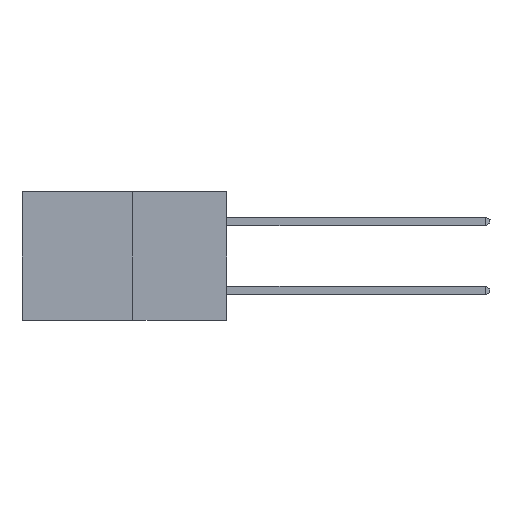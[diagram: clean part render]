
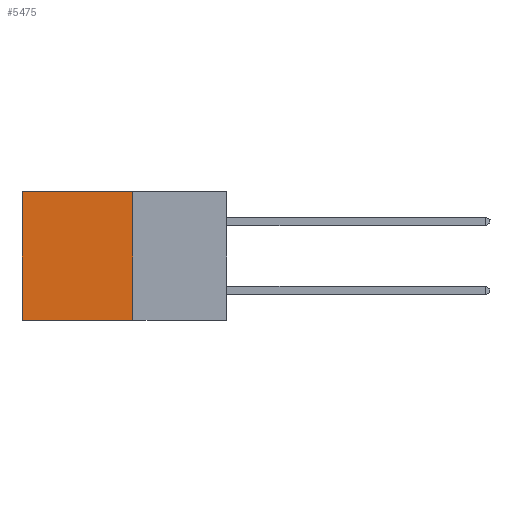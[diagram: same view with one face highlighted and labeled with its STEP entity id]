
A CAD part, left-side view. The second image highlights one B-rep face of the part: STEP entity #5475.
In plain terms, the highlighted planar face has unit normal (-1, 0, 0).
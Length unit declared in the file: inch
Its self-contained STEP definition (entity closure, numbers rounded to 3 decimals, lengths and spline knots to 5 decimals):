
#87 = AXIS2_PLACEMENT_3D ( 'NONE', #12365, #12074, #12022 ) ;
#918 = CARTESIAN_POINT ( 'NONE',  ( 0.277, 0.27, -0.37 ) ) ;
#1489 = CARTESIAN_POINT ( 'NONE',  ( 0.277, 0.27, 0. ) ) ;
#1579 = VERTEX_POINT ( 'NONE', #26224 ) ;
#1905 = ORIENTED_EDGE ( 'NONE', *, *, #10503, .T. ) ;
#2034 = FACE_OUTER_BOUND ( 'NONE', #7425, .T. ) ;
#2120 = CARTESIAN_POINT ( 'NONE',  ( 0.277, 0.27, -0.37 ) ) ;
#5475 = ADVANCED_FACE ( 'NONE', ( #2034 ), #12141, .F. ) ;
#6889 = LINE ( 'NONE', #16978, #12158 ) ;
#7425 = EDGE_LOOP ( 'NONE', ( #1905, #21946, #28570, #7823 ) ) ;
#7705 = CARTESIAN_POINT ( 'NONE',  ( 0.277, 0.59, -0.37 ) ) ;
#7823 = ORIENTED_EDGE ( 'NONE', *, *, #11074, .T. ) ;
#9882 = LINE ( 'NONE', #2120, #15215 ) ;
#10503 = EDGE_CURVE ( 'NONE', #19440, #12695, #6889, .T. ) ;
#11074 = EDGE_CURVE ( 'NONE', #1579, #19440, #13713, .T. ) ;
#11922 = DIRECTION ( 'NONE',  ( 0., 0., -1. ) ) ;
#12022 = DIRECTION ( 'NONE',  ( 0., 0., -1. ) ) ;
#12074 = DIRECTION ( 'NONE',  ( 1., 0., 0. ) ) ;
#12141 = PLANE ( 'NONE',  #87 ) ;
#12158 = VECTOR ( 'NONE', #12417, 39.37008 ) ;
#12365 = CARTESIAN_POINT ( 'NONE',  ( 0.277, 0.27, -0.37 ) ) ;
#12417 = DIRECTION ( 'NONE',  ( 0., 0., -1. ) ) ;
#12695 = VERTEX_POINT ( 'NONE', #7705 ) ;
#12770 = CARTESIAN_POINT ( 'NONE',  ( 0.277, 0.59, 0. ) ) ;
#13526 = DIRECTION ( 'NONE',  ( 0., 1., 0. ) ) ;
#13713 = LINE ( 'NONE', #1489, #18988 ) ;
#15212 = DIRECTION ( 'NONE',  ( 0., 1., 0. ) ) ;
#15215 = VECTOR ( 'NONE', #13526, 39.37008 ) ;
#16978 = CARTESIAN_POINT ( 'NONE',  ( 0.277, 0.59, -0.37 ) ) ;
#18988 = VECTOR ( 'NONE', #15212, 39.37008 ) ;
#19149 = VECTOR ( 'NONE', #11922, 39.37008 ) ;
#19318 = VERTEX_POINT ( 'NONE', #918 ) ;
#19440 = VERTEX_POINT ( 'NONE', #12770 ) ;
#21946 = ORIENTED_EDGE ( 'NONE', *, *, #22121, .F. ) ;
#22121 = EDGE_CURVE ( 'NONE', #19318, #12695, #9882, .T. ) ;
#23209 = CARTESIAN_POINT ( 'NONE',  ( 0.277, 0.27, -0.37 ) ) ;
#25184 = LINE ( 'NONE', #23209, #19149 ) ;
#26224 = CARTESIAN_POINT ( 'NONE',  ( 0.277, 0.27, 0. ) ) ;
#27914 = EDGE_CURVE ( 'NONE', #1579, #19318, #25184, .T. ) ;
#28570 = ORIENTED_EDGE ( 'NONE', *, *, #27914, .F. ) ;
